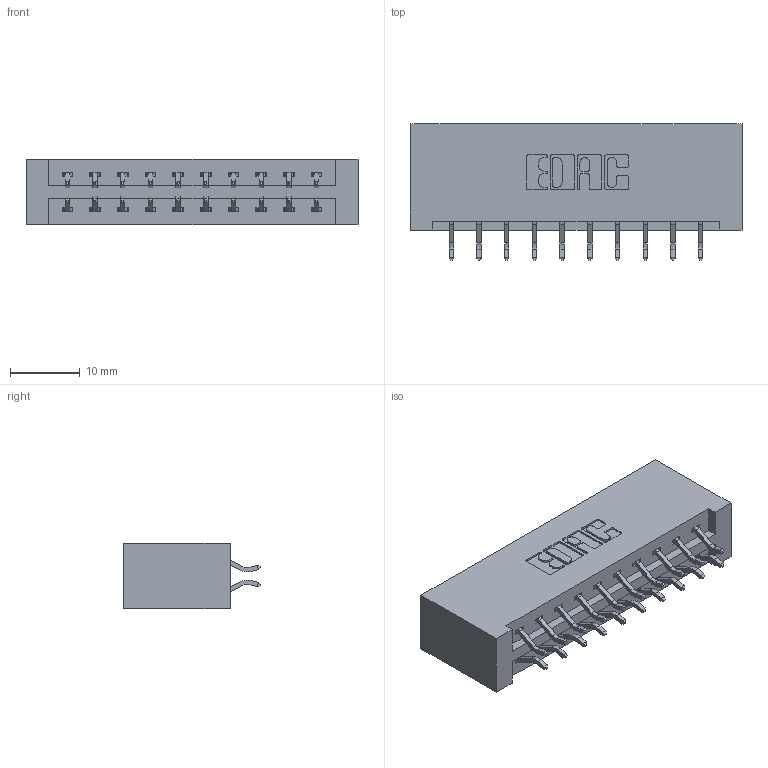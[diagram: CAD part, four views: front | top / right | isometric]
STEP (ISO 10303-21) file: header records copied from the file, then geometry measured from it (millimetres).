
FILE_DESCRIPTION (( 'STEP AP203' ), '1' );
FILE_NAME ('387-020-556-201.STEP', '2019-10-16T15:49:59', ( '' ), ( '' ), 'SwSTEP 2.0', 'SolidWorks 2016', '' );
FILE_SCHEMA (( 'CONFIG_CONTROL_DESIGN' ));
Length unit declared in the file: inch
Products named in the file (3): 345-292-001_556 Tail; 387-020-556-201; 337 Part_No Mounting Lugs
Assembly tree (21 placements, depth 2):
  387-020-556-201
    337 Part_No Mounting Lugs
    345-292-001_556 Tail  x20
Bounding box: 47.5 x 19.57 x 9.4 mm (x, y, z)
Volume: 5339.7 mm3; surface area: 5760.7 mm2
Topology: 21 solids, 21 shells, 1306 faces, 3867 edges, 2550 vertices
Faces by surface type: plane 906, cylinder 400
Entity records: 11835 total; most frequent: CARTESIAN_POINT 2034, ORIENTED_EDGE 1958, DIRECTION 1771, EDGE_CURVE 979, LINE 851, VECTOR 851, VERTEX_POINT 650, AXIS2_PLACEMENT_3D 460
